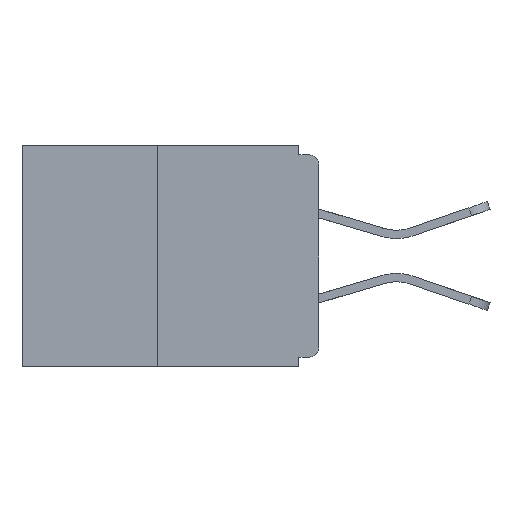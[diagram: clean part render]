
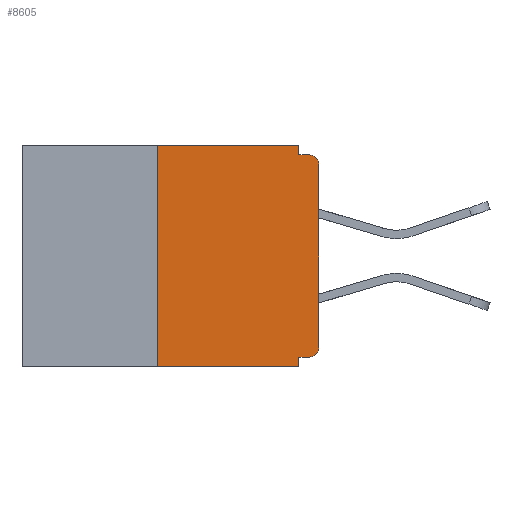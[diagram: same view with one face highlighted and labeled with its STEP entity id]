
A CAD part, left-side view. The second image highlights one B-rep face of the part: STEP entity #8605.
In plain terms, the highlighted planar face has unit normal (-1, 0, 0).
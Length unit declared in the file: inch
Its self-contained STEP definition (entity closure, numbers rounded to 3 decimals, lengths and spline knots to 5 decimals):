
#87 = CARTESIAN_POINT ( 'NONE',  ( 0., 0.031, 0. ) ) ;
#127 = DIRECTION ( 'NONE',  ( 0., 0., 1. ) ) ;
#598 = AXIS2_PLACEMENT_3D ( 'NONE', #11486, #10125, #3430 ) ;
#738 = EDGE_CURVE ( 'NONE', #8581, #9583, #6956, .T. ) ;
#1214 = DIRECTION ( 'NONE',  ( -1., 0., 0. ) ) ;
#1403 = LINE ( 'NONE', #11739, #3299 ) ;
#1726 = CARTESIAN_POINT ( 'NONE',  ( 0., 0.46, 0. ) ) ;
#1806 = CARTESIAN_POINT ( 'NONE',  ( 0., 0.031, -0.015 ) ) ;
#1948 = DIRECTION ( 'NONE',  ( 0., 0., -1. ) ) ;
#2039 = DIRECTION ( 'NONE',  ( 0., -1., 0. ) ) ;
#2647 = EDGE_CURVE ( 'NONE', #14276, #9583, #11383, .T. ) ;
#2927 = EDGE_CURVE ( 'NONE', #15101, #14276, #1403, .T. ) ;
#3247 = ORIENTED_EDGE ( 'NONE', *, *, #2927, .T. ) ;
#3299 = VECTOR ( 'NONE', #127, 39.37008 ) ;
#3430 = DIRECTION ( 'NONE',  ( 0., 0., -1. ) ) ;
#3442 = EDGE_CURVE ( 'NONE', #4056, #6834, #5702, .T. ) ;
#3565 = EDGE_CURVE ( 'NONE', #5039, #14289, #3642, .T. ) ;
#3642 = LINE ( 'NONE', #16195, #5101 ) ;
#3999 = ORIENTED_EDGE ( 'NONE', *, *, #4591, .T. ) ;
#4056 = VERTEX_POINT ( 'NONE', #11668 ) ;
#4128 = DIRECTION ( 'NONE',  ( 0., 1., 0. ) ) ;
#4229 = EDGE_LOOP ( 'NONE', ( #6898, #16550, #3999, #9699, #4295, #11287, #3247, #7452, #5105, #15604 ) ) ;
#4295 = ORIENTED_EDGE ( 'NONE', *, *, #9248, .F. ) ;
#4362 = DIRECTION ( 'NONE',  ( 0., 0., -1. ) ) ;
#4591 = EDGE_CURVE ( 'NONE', #16458, #6834, #5111, .T. ) ;
#4654 = LINE ( 'NONE', #11180, #10307 ) ;
#5039 = VERTEX_POINT ( 'NONE', #14146 ) ;
#5077 = DIRECTION ( 'NONE',  ( 0., 0., 1. ) ) ;
#5101 = VECTOR ( 'NONE', #2039, 39.37008 ) ;
#5105 = ORIENTED_EDGE ( 'NONE', *, *, #738, .F. ) ;
#5111 = LINE ( 'NONE', #9164, #11466 ) ;
#5223 = AXIS2_PLACEMENT_3D ( 'NONE', #6651, #1214, #14442 ) ;
#5702 = LINE ( 'NONE', #6971, #13263 ) ;
#6480 = DIRECTION ( 'NONE',  ( 0., -1., 0. ) ) ;
#6651 = CARTESIAN_POINT ( 'NONE',  ( 0., 0.015, -0.313 ) ) ;
#6672 = LINE ( 'NONE', #11822, #12668 ) ;
#6834 = VERTEX_POINT ( 'NONE', #8273 ) ;
#6898 = ORIENTED_EDGE ( 'NONE', *, *, #3565, .F. ) ;
#6956 = LINE ( 'NONE', #13223, #13177 ) ;
#6971 = CARTESIAN_POINT ( 'NONE',  ( 0., 0.031, -0.343 ) ) ;
#6983 = PLANE ( 'NONE',  #13778 ) ;
#7452 = ORIENTED_EDGE ( 'NONE', *, *, #2647, .T. ) ;
#8273 = CARTESIAN_POINT ( 'NONE',  ( 0., 0.031, -0.343 ) ) ;
#8581 = VERTEX_POINT ( 'NONE', #1806 ) ;
#8605 = ADVANCED_FACE ( 'NONE', ( #13083 ), #6983, .F. ) ;
#8723 = CARTESIAN_POINT ( 'NONE',  ( 0., 0.25, -0.343 ) ) ;
#8793 = CARTESIAN_POINT ( 'NONE',  ( 0., 0., -0.03 ) ) ;
#9164 = CARTESIAN_POINT ( 'NONE',  ( 0., 0.46, -0.343 ) ) ;
#9248 = EDGE_CURVE ( 'NONE', #15835, #4056, #6672, .T. ) ;
#9258 = CIRCLE ( 'NONE', #5223, 0.015 ) ;
#9262 = DIRECTION ( 'NONE',  ( 1., 0., 0. ) ) ;
#9583 = VERTEX_POINT ( 'NONE', #11394 ) ;
#9699 = ORIENTED_EDGE ( 'NONE', *, *, #3442, .F. ) ;
#10125 = DIRECTION ( 'NONE',  ( -1., 0., 0. ) ) ;
#10307 = VECTOR ( 'NONE', #1948, 39.37008 ) ;
#10409 = EDGE_CURVE ( 'NONE', #16458, #5039, #11603, .T. ) ;
#11079 = VECTOR ( 'NONE', #5077, 39.37008 ) ;
#11180 = CARTESIAN_POINT ( 'NONE',  ( 0., 0.031, 0. ) ) ;
#11287 = ORIENTED_EDGE ( 'NONE', *, *, #13403, .T. ) ;
#11383 = CIRCLE ( 'NONE', #598, 0.015 ) ;
#11394 = CARTESIAN_POINT ( 'NONE',  ( 0., 0.015, -0.015 ) ) ;
#11466 = VECTOR ( 'NONE', #6480, 39.37008 ) ;
#11486 = CARTESIAN_POINT ( 'NONE',  ( 0., 0.015, -0.03 ) ) ;
#11603 = LINE ( 'NONE', #14157, #11079 ) ;
#11668 = CARTESIAN_POINT ( 'NONE',  ( 0., 0.031, -0.328 ) ) ;
#11739 = CARTESIAN_POINT ( 'NONE',  ( 0., 0., 0. ) ) ;
#11822 = CARTESIAN_POINT ( 'NONE',  ( 0., 0., -0.328 ) ) ;
#11839 = EDGE_CURVE ( 'NONE', #14289, #8581, #4654, .T. ) ;
#12668 = VECTOR ( 'NONE', #4128, 39.37008 ) ;
#12933 = CARTESIAN_POINT ( 'NONE',  ( 0., 0.015, -0.328 ) ) ;
#13083 = FACE_OUTER_BOUND ( 'NONE', #4229, .T. ) ;
#13177 = VECTOR ( 'NONE', #13320, 39.37008 ) ;
#13223 = CARTESIAN_POINT ( 'NONE',  ( 0., 0., -0.015 ) ) ;
#13263 = VECTOR ( 'NONE', #14844, 39.37008 ) ;
#13320 = DIRECTION ( 'NONE',  ( 0., -1., 0. ) ) ;
#13403 = EDGE_CURVE ( 'NONE', #15835, #15101, #9258, .T. ) ;
#13778 = AXIS2_PLACEMENT_3D ( 'NONE', #1726, #9262, #4362 ) ;
#14146 = CARTESIAN_POINT ( 'NONE',  ( 0., 0.25, 0. ) ) ;
#14157 = CARTESIAN_POINT ( 'NONE',  ( 0., 0.25, 0. ) ) ;
#14276 = VERTEX_POINT ( 'NONE', #8793 ) ;
#14289 = VERTEX_POINT ( 'NONE', #87 ) ;
#14442 = DIRECTION ( 'NONE',  ( 0., 0., -1. ) ) ;
#14580 = CARTESIAN_POINT ( 'NONE',  ( 0., 0., -0.313 ) ) ;
#14844 = DIRECTION ( 'NONE',  ( 0., 0., -1. ) ) ;
#15101 = VERTEX_POINT ( 'NONE', #14580 ) ;
#15604 = ORIENTED_EDGE ( 'NONE', *, *, #11839, .F. ) ;
#15835 = VERTEX_POINT ( 'NONE', #12933 ) ;
#16195 = CARTESIAN_POINT ( 'NONE',  ( 0., 0.46, 0. ) ) ;
#16458 = VERTEX_POINT ( 'NONE', #8723 ) ;
#16550 = ORIENTED_EDGE ( 'NONE', *, *, #10409, .F. ) ;
